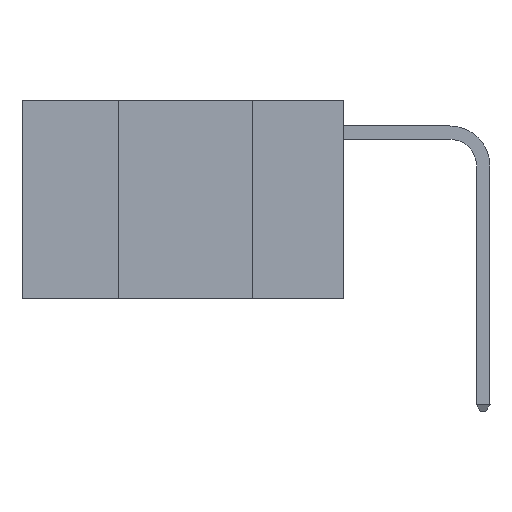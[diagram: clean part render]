
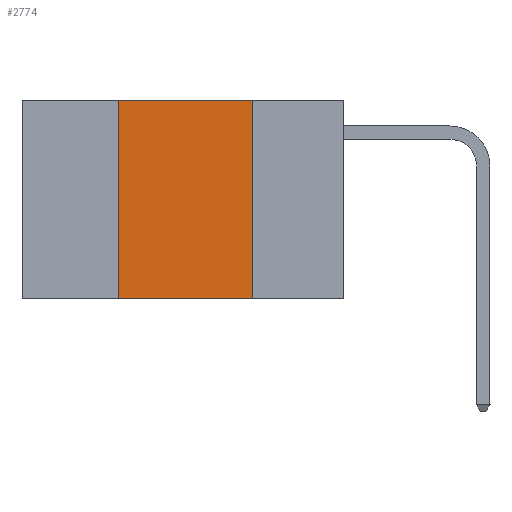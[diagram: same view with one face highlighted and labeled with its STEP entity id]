
A CAD part, left-side view. The second image highlights one B-rep face of the part: STEP entity #2774.
In plain terms, the highlighted planar face has unit normal (-1, 0, 0).
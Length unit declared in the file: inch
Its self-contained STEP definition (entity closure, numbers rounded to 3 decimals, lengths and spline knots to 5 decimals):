
#48 = EDGE_CURVE ( 'NONE', #13010, #14944, #4596, .T. ) ;
#345 = ORIENTED_EDGE ( 'NONE', *, *, #15056, .F. ) ;
#1055 = CARTESIAN_POINT ( 'NONE',  ( 0., 0.42, -0.37 ) ) ;
#1069 = AXIS2_PLACEMENT_3D ( 'NONE', #10191, #4172, #12837 ) ;
#1353 = VECTOR ( 'NONE', #14448, 39.37008 ) ;
#2774 = ADVANCED_FACE ( 'NONE', ( #9128 ), #12957, .F. ) ;
#3117 = DIRECTION ( 'NONE',  ( 0., -1., 0. ) ) ;
#3420 = EDGE_CURVE ( 'NONE', #14944, #6875, #11135, .T. ) ;
#4003 = VECTOR ( 'NONE', #3117, 39.37008 ) ;
#4172 = DIRECTION ( 'NONE',  ( 1., 0., 0. ) ) ;
#4596 = LINE ( 'NONE', #14492, #1353 ) ;
#5950 = CARTESIAN_POINT ( 'NONE',  ( 0., 0.17, 0. ) ) ;
#6422 = VERTEX_POINT ( 'NONE', #11702 ) ;
#6695 = VECTOR ( 'NONE', #13810, 39.37008 ) ;
#6875 = VERTEX_POINT ( 'NONE', #9028 ) ;
#7073 = CARTESIAN_POINT ( 'NONE',  ( 0., 0.42, 0. ) ) ;
#7649 = EDGE_CURVE ( 'NONE', #13010, #6422, #8336, .T. ) ;
#7653 = ORIENTED_EDGE ( 'NONE', *, *, #3420, .F. ) ;
#8071 = ORIENTED_EDGE ( 'NONE', *, *, #48, .F. ) ;
#8336 = LINE ( 'NONE', #14313, #14843 ) ;
#8926 = EDGE_LOOP ( 'NONE', ( #345, #7653, #8071, #14987 ) ) ;
#9028 = CARTESIAN_POINT ( 'NONE',  ( 0., 0.17, 0. ) ) ;
#9128 = FACE_OUTER_BOUND ( 'NONE', #8926, .T. ) ;
#10191 = CARTESIAN_POINT ( 'NONE',  ( 0., 0.6, 0. ) ) ;
#10250 = LINE ( 'NONE', #5950, #6695 ) ;
#11135 = LINE ( 'NONE', #13597, #4003 ) ;
#11702 = CARTESIAN_POINT ( 'NONE',  ( 0., 0.17, -0.37 ) ) ;
#11727 = DIRECTION ( 'NONE',  ( 0., -1., 0. ) ) ;
#12837 = DIRECTION ( 'NONE',  ( 0., 0., -1. ) ) ;
#12957 = PLANE ( 'NONE',  #1069 ) ;
#13010 = VERTEX_POINT ( 'NONE', #1055 ) ;
#13597 = CARTESIAN_POINT ( 'NONE',  ( 0., 0.6, 0. ) ) ;
#13810 = DIRECTION ( 'NONE',  ( 0., 0., -1. ) ) ;
#14313 = CARTESIAN_POINT ( 'NONE',  ( 0., 0.6, -0.37 ) ) ;
#14448 = DIRECTION ( 'NONE',  ( 0., 0., 1. ) ) ;
#14492 = CARTESIAN_POINT ( 'NONE',  ( 0., 0.42, 0. ) ) ;
#14843 = VECTOR ( 'NONE', #11727, 39.37008 ) ;
#14944 = VERTEX_POINT ( 'NONE', #7073 ) ;
#14987 = ORIENTED_EDGE ( 'NONE', *, *, #7649, .T. ) ;
#15056 = EDGE_CURVE ( 'NONE', #6875, #6422, #10250, .T. ) ;
